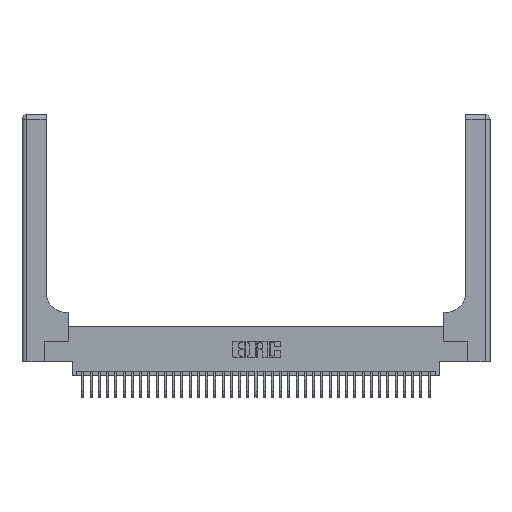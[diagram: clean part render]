
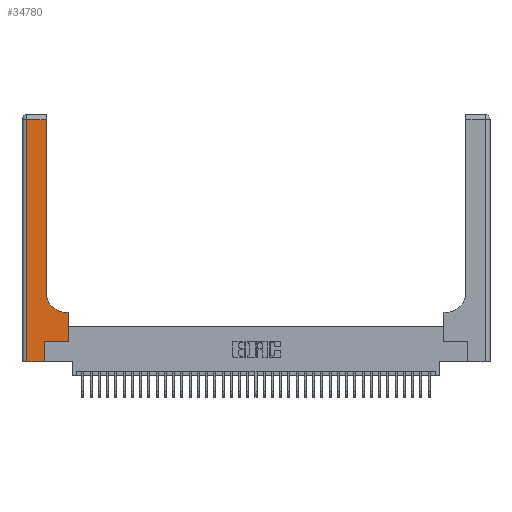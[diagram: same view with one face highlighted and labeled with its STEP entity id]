
A CAD part, top view. The second image highlights one B-rep face of the part: STEP entity #34780.
In plain terms, the highlighted planar face has unit normal (0, 0, 1).
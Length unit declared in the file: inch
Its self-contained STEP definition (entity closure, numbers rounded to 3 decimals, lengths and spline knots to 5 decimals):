
#54 = DIRECTION ( 'NONE',  ( 1., 0., 0. ) ) ;
#282 = VERTEX_POINT ( 'NONE', #36264 ) ;
#699 = CARTESIAN_POINT ( 'NONE',  ( 0.5585, 0.6, 0.37 ) ) ;
#1245 = VERTEX_POINT ( 'NONE', #16469 ) ;
#1821 = VECTOR ( 'NONE', #28475, 39.37008 ) ;
#1956 = DIRECTION ( 'NONE',  ( -1., 0., 0. ) ) ;
#2352 = LINE ( 'NONE', #36626, #18224 ) ;
#2823 = VECTOR ( 'NONE', #34161, 39.37008 ) ;
#2904 = VERTEX_POINT ( 'NONE', #11375 ) ;
#5324 = LINE ( 'NONE', #24465, #30400 ) ;
#5559 = DIRECTION ( 'NONE',  ( 1., 0., 0. ) ) ;
#5595 = DIRECTION ( 'NONE',  ( 0., 1., 0. ) ) ;
#5629 = CIRCLE ( 'NONE', #13502, 0.25 ) ;
#5952 = CARTESIAN_POINT ( 'NONE',  ( 0., 0., 0.37 ) ) ;
#6369 = VERTEX_POINT ( 'NONE', #33487 ) ;
#6504 = CARTESIAN_POINT ( 'NONE',  ( 0., 2.94, 0.37 ) ) ;
#7557 = VECTOR ( 'NONE', #23205, 39.37008 ) ;
#8849 = ORIENTED_EDGE ( 'NONE', *, *, #22549, .T. ) ;
#9409 = EDGE_LOOP ( 'NONE', ( #25124, #30514, #22424, #38052, #16819, #8849, #11990, #35449, #21412 ) ) ;
#10252 = LINE ( 'NONE', #31645, #25963 ) ;
#10357 = CARTESIAN_POINT ( 'NONE',  ( 0.06, 3., 0.37 ) ) ;
#11375 = CARTESIAN_POINT ( 'NONE',  ( 0.06, 2.94, 0.37 ) ) ;
#11990 = ORIENTED_EDGE ( 'NONE', *, *, #12220, .T. ) ;
#12220 = EDGE_CURVE ( 'NONE', #282, #25000, #2352, .T. ) ;
#12469 = EDGE_CURVE ( 'NONE', #6369, #2904, #17730, .T. ) ;
#12748 = VERTEX_POINT ( 'NONE', #26562 ) ;
#12927 = DIRECTION ( 'NONE',  ( 0., 1., 0. ) ) ;
#13502 = AXIS2_PLACEMENT_3D ( 'NONE', #37630, #19047, #54 ) ;
#13555 = DIRECTION ( 'NONE',  ( 0., -1., 0. ) ) ;
#14608 = PLANE ( 'NONE',  #20047 ) ;
#14853 = DIRECTION ( 'NONE',  ( 0., 1., 0. ) ) ;
#15033 = VERTEX_POINT ( 'NONE', #36127 ) ;
#15177 = EDGE_CURVE ( 'NONE', #12748, #6369, #5324, .T. ) ;
#16469 = CARTESIAN_POINT ( 'NONE',  ( 0.06, 0., 0.37 ) ) ;
#16819 = ORIENTED_EDGE ( 'NONE', *, *, #40522, .T. ) ;
#16938 = CARTESIAN_POINT ( 'NONE',  ( 0.2915, 0.6, 0.37 ) ) ;
#17730 = LINE ( 'NONE', #6504, #1821 ) ;
#18224 = VECTOR ( 'NONE', #14853, 39.37008 ) ;
#18926 = CARTESIAN_POINT ( 'NONE',  ( 0.269, 0., 0.37 ) ) ;
#18941 = FACE_OUTER_BOUND ( 'NONE', #9409, .T. ) ;
#19047 = DIRECTION ( 'NONE',  ( 0., 0., -1. ) ) ;
#20047 = AXIS2_PLACEMENT_3D ( 'NONE', #30179, #20918, #1956 ) ;
#20227 = EDGE_CURVE ( 'NONE', #25000, #15033, #24314, .T. ) ;
#20489 = CARTESIAN_POINT ( 'NONE',  ( 0.269, 0.25, 0.37 ) ) ;
#20918 = DIRECTION ( 'NONE',  ( 0., 0., -1. ) ) ;
#21412 = ORIENTED_EDGE ( 'NONE', *, *, #26604, .T. ) ;
#22424 = ORIENTED_EDGE ( 'NONE', *, *, #31481, .T. ) ;
#22549 = EDGE_CURVE ( 'NONE', #32273, #282, #40605, .T. ) ;
#22943 = VECTOR ( 'NONE', #13555, 39.37008 ) ;
#23205 = DIRECTION ( 'NONE',  ( -1., 0., 0. ) ) ;
#24060 = EDGE_CURVE ( 'NONE', #1245, #26829, #27943, .T. ) ;
#24314 = LINE ( 'NONE', #16938, #7557 ) ;
#24465 = CARTESIAN_POINT ( 'NONE',  ( 0.2915, 3., 0.37 ) ) ;
#25000 = VERTEX_POINT ( 'NONE', #699 ) ;
#25124 = ORIENTED_EDGE ( 'NONE', *, *, #15177, .T. ) ;
#25963 = VECTOR ( 'NONE', #12927, 39.37008 ) ;
#26562 = CARTESIAN_POINT ( 'NONE',  ( 0.2915, 0.85, 0.37 ) ) ;
#26604 = EDGE_CURVE ( 'NONE', #15033, #12748, #5629, .T. ) ;
#26829 = VERTEX_POINT ( 'NONE', #18926 ) ;
#27943 = LINE ( 'NONE', #5952, #2823 ) ;
#28475 = DIRECTION ( 'NONE',  ( -1., 0., 0. ) ) ;
#30179 = CARTESIAN_POINT ( 'NONE',  ( 0., 3., 0.37 ) ) ;
#30400 = VECTOR ( 'NONE', #5595, 39.37008 ) ;
#30514 = ORIENTED_EDGE ( 'NONE', *, *, #12469, .T. ) ;
#31481 = EDGE_CURVE ( 'NONE', #2904, #1245, #32177, .T. ) ;
#31645 = CARTESIAN_POINT ( 'NONE',  ( 0.269, 0., 0.37 ) ) ;
#32177 = LINE ( 'NONE', #10357, #22943 ) ;
#32273 = VERTEX_POINT ( 'NONE', #20489 ) ;
#32356 = VECTOR ( 'NONE', #5559, 39.37008 ) ;
#33487 = CARTESIAN_POINT ( 'NONE',  ( 0.2915, 2.94, 0.37 ) ) ;
#34161 = DIRECTION ( 'NONE',  ( 1., 0., 0. ) ) ;
#34780 = ADVANCED_FACE ( 'NONE', ( #18941 ), #14608, .F. ) ;
#35449 = ORIENTED_EDGE ( 'NONE', *, *, #20227, .T. ) ;
#36127 = CARTESIAN_POINT ( 'NONE',  ( 0.5415, 0.6, 0.37 ) ) ;
#36264 = CARTESIAN_POINT ( 'NONE',  ( 0.5585, 0.25, 0.37 ) ) ;
#36626 = CARTESIAN_POINT ( 'NONE',  ( 0.5585, 0.25, 0.37 ) ) ;
#36759 = CARTESIAN_POINT ( 'NONE',  ( 0.269, 0.25, 0.37 ) ) ;
#37630 = CARTESIAN_POINT ( 'NONE',  ( 0.5415, 0.85, 0.37 ) ) ;
#38052 = ORIENTED_EDGE ( 'NONE', *, *, #24060, .T. ) ;
#40522 = EDGE_CURVE ( 'NONE', #26829, #32273, #10252, .T. ) ;
#40605 = LINE ( 'NONE', #36759, #32356 ) ;
